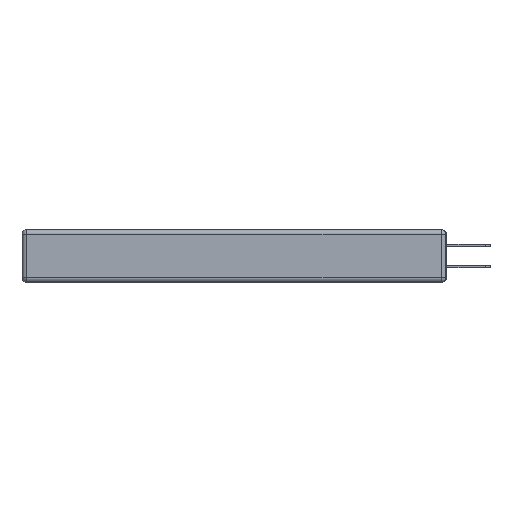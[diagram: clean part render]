
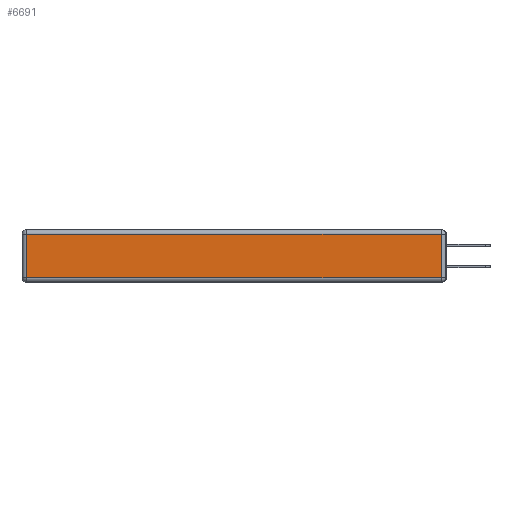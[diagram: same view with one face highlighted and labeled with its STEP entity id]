
A CAD part, left-side view. The second image highlights one B-rep face of the part: STEP entity #6691.
In plain terms, the highlighted planar face has unit normal (-1, 0, 0).
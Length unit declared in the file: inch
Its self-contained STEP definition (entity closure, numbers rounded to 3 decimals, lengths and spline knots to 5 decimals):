
#645 = PLANE ( 'NONE',  #5054 ) ;
#1265 = EDGE_CURVE ( 'NONE', #1679, #10131, #17493, .T. ) ;
#1679 = VERTEX_POINT ( 'NONE', #3311 ) ;
#3150 = DIRECTION ( 'NONE',  ( 0., 1., 0. ) ) ;
#3294 = DIRECTION ( 'NONE',  ( -1., 0., 0. ) ) ;
#3311 = CARTESIAN_POINT ( 'NONE',  ( 0., 0.03, -0.03 ) ) ;
#3466 = ORIENTED_EDGE ( 'NONE', *, *, #10385, .T. ) ;
#3541 = VERTEX_POINT ( 'NONE', #14238 ) ;
#4110 = LINE ( 'NONE', #17163, #4752 ) ;
#4512 = VECTOR ( 'NONE', #3150, 39.37008 ) ;
#4568 = CARTESIAN_POINT ( 'NONE',  ( 0., 0., -0.343 ) ) ;
#4752 = VECTOR ( 'NONE', #9062, 39.37008 ) ;
#5054 = AXIS2_PLACEMENT_3D ( 'NONE', #4568, #3294, #12765 ) ;
#5241 = CARTESIAN_POINT ( 'NONE',  ( 0., 2.72, -0.03 ) ) ;
#5484 = ORIENTED_EDGE ( 'NONE', *, *, #1265, .T. ) ;
#5733 = VECTOR ( 'NONE', #16759, 39.37008 ) ;
#6691 = ADVANCED_FACE ( 'NONE', ( #13116 ), #645, .T. ) ;
#6833 = CARTESIAN_POINT ( 'NONE',  ( 0., 2.72, -0.343 ) ) ;
#7159 = VERTEX_POINT ( 'NONE', #8143 ) ;
#7232 = ORIENTED_EDGE ( 'NONE', *, *, #12984, .T. ) ;
#8143 = CARTESIAN_POINT ( 'NONE',  ( 0., 2.72, -0.313 ) ) ;
#8254 = DIRECTION ( 'NONE',  ( 0., 0., -1. ) ) ;
#8748 = CARTESIAN_POINT ( 'NONE',  ( 0., 0.03, -0.343 ) ) ;
#8826 = ORIENTED_EDGE ( 'NONE', *, *, #9228, .T. ) ;
#9062 = DIRECTION ( 'NONE',  ( 0., -1., 0. ) ) ;
#9228 = EDGE_CURVE ( 'NONE', #10131, #7159, #13435, .T. ) ;
#10001 = LINE ( 'NONE', #8748, #5733 ) ;
#10131 = VERTEX_POINT ( 'NONE', #5241 ) ;
#10176 = EDGE_LOOP ( 'NONE', ( #7232, #3466, #5484, #8826 ) ) ;
#10385 = EDGE_CURVE ( 'NONE', #3541, #1679, #10001, .T. ) ;
#12765 = DIRECTION ( 'NONE',  ( 0., 0., 1. ) ) ;
#12984 = EDGE_CURVE ( 'NONE', #7159, #3541, #4110, .T. ) ;
#13116 = FACE_OUTER_BOUND ( 'NONE', #10176, .T. ) ;
#13435 = LINE ( 'NONE', #6833, #16419 ) ;
#14238 = CARTESIAN_POINT ( 'NONE',  ( 0., 0.03, -0.313 ) ) ;
#16419 = VECTOR ( 'NONE', #8254, 39.37008 ) ;
#16729 = CARTESIAN_POINT ( 'NONE',  ( 0., 2.75, -0.03 ) ) ;
#16759 = DIRECTION ( 'NONE',  ( 0., 0., 1. ) ) ;
#17163 = CARTESIAN_POINT ( 'NONE',  ( 0., 0., -0.313 ) ) ;
#17493 = LINE ( 'NONE', #16729, #4512 ) ;
